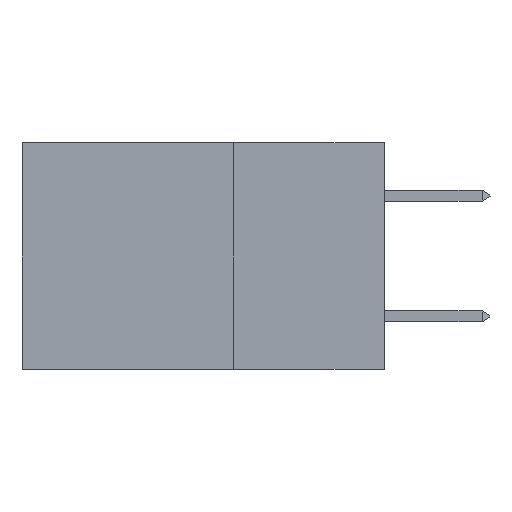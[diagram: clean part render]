
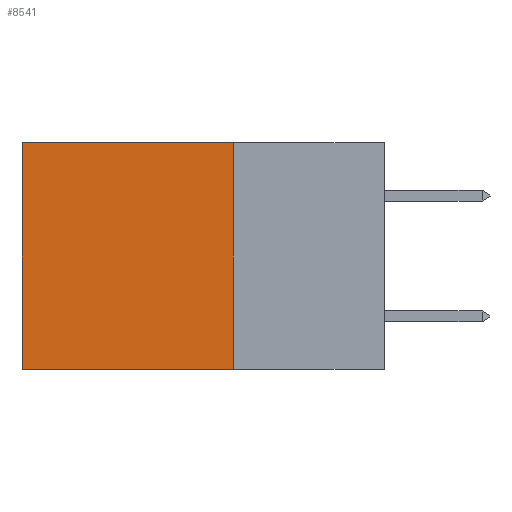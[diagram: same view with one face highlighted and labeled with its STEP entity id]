
A CAD part, left-side view. The second image highlights one B-rep face of the part: STEP entity #8541.
In plain terms, the highlighted planar face has unit normal (-1, 0, 0).
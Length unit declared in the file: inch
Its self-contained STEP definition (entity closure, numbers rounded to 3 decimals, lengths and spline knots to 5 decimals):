
#733 = LINE ( 'NONE', #2000, #3677 ) ;
#1273 = EDGE_CURVE ( 'NONE', #7046, #7253, #6593, .T. ) ;
#1910 = VECTOR ( 'NONE', #14620, 39.37008 ) ;
#1915 = CARTESIAN_POINT ( 'NONE',  ( 0.2875, 0.25, -0.375 ) ) ;
#2000 = CARTESIAN_POINT ( 'NONE',  ( 0.2875, 0.25, -0.375 ) ) ;
#2912 = PLANE ( 'NONE',  #10711 ) ;
#3123 = VECTOR ( 'NONE', #3309, 39.37008 ) ;
#3309 = DIRECTION ( 'NONE',  ( 0., 0., -1. ) ) ;
#3601 = CARTESIAN_POINT ( 'NONE',  ( 0.2875, 0.6, 0. ) ) ;
#3677 = VECTOR ( 'NONE', #5342, 39.37008 ) ;
#4228 = EDGE_LOOP ( 'NONE', ( #10879, #4859, #7680, #13106 ) ) ;
#4533 = VERTEX_POINT ( 'NONE', #6036 ) ;
#4859 = ORIENTED_EDGE ( 'NONE', *, *, #6955, .F. ) ;
#5108 = FACE_OUTER_BOUND ( 'NONE', #4228, .T. ) ;
#5342 = DIRECTION ( 'NONE',  ( 0., 1., 0. ) ) ;
#5351 = CARTESIAN_POINT ( 'NONE',  ( 0.2875, 0.25, 0. ) ) ;
#6036 = CARTESIAN_POINT ( 'NONE',  ( 0.2875, 0.6, -0.375 ) ) ;
#6156 = DIRECTION ( 'NONE',  ( 0., 0., -1. ) ) ;
#6593 = LINE ( 'NONE', #10089, #12448 ) ;
#6955 = EDGE_CURVE ( 'NONE', #7253, #4533, #733, .T. ) ;
#7046 = VERTEX_POINT ( 'NONE', #7151 ) ;
#7151 = CARTESIAN_POINT ( 'NONE',  ( 0.2875, 0.25, 0. ) ) ;
#7253 = VERTEX_POINT ( 'NONE', #1915 ) ;
#7288 = DIRECTION ( 'NONE',  ( 1., 0., 0. ) ) ;
#7680 = ORIENTED_EDGE ( 'NONE', *, *, #1273, .F. ) ;
#8541 = ADVANCED_FACE ( 'NONE', ( #5108 ), #2912, .F. ) ;
#9591 = VERTEX_POINT ( 'NONE', #3601 ) ;
#9728 = CARTESIAN_POINT ( 'NONE',  ( 0.2875, 0.25, -0.375 ) ) ;
#10089 = CARTESIAN_POINT ( 'NONE',  ( 0.2875, 0.25, -0.375 ) ) ;
#10711 = AXIS2_PLACEMENT_3D ( 'NONE', #9728, #7288, #6156 ) ;
#10727 = EDGE_CURVE ( 'NONE', #9591, #4533, #13701, .T. ) ;
#10879 = ORIENTED_EDGE ( 'NONE', *, *, #10727, .T. ) ;
#11116 = LINE ( 'NONE', #5351, #1910 ) ;
#11954 = EDGE_CURVE ( 'NONE', #7046, #9591, #11116, .T. ) ;
#12448 = VECTOR ( 'NONE', #14882, 39.37008 ) ;
#13106 = ORIENTED_EDGE ( 'NONE', *, *, #11954, .T. ) ;
#13701 = LINE ( 'NONE', #14773, #3123 ) ;
#14620 = DIRECTION ( 'NONE',  ( 0., 1., 0. ) ) ;
#14773 = CARTESIAN_POINT ( 'NONE',  ( 0.2875, 0.6, -0.375 ) ) ;
#14882 = DIRECTION ( 'NONE',  ( 0., 0., -1. ) ) ;
